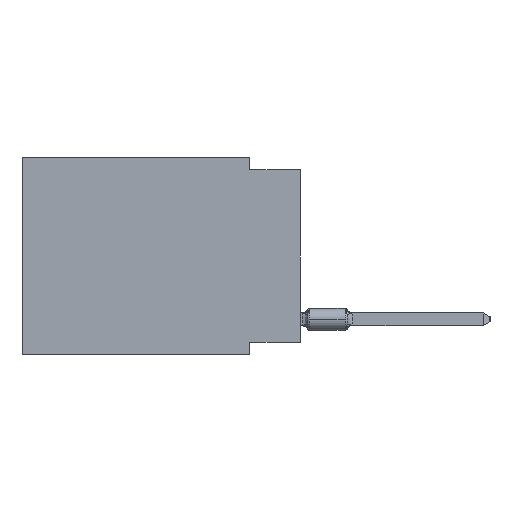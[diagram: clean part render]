
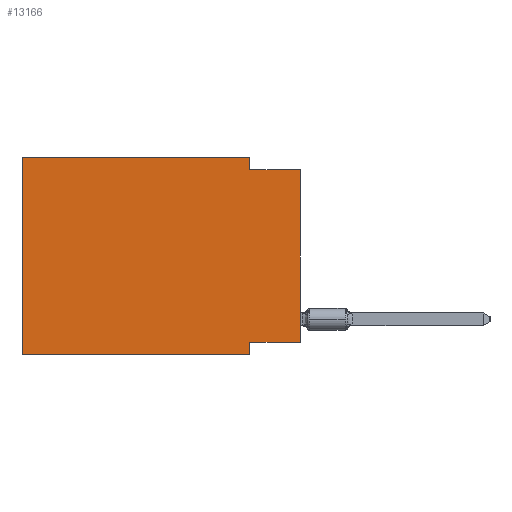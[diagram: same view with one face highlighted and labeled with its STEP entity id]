
A CAD part, left-side view. The second image highlights one B-rep face of the part: STEP entity #13166.
In plain terms, the highlighted planar face has unit normal (-1, 0, 0).
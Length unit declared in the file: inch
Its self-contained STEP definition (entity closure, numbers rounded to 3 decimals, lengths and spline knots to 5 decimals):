
#811 = CARTESIAN_POINT ( 'NONE',  ( 0., 0.1, -0.39 ) ) ;
#1030 = FACE_OUTER_BOUND ( 'NONE', #21980, .T. ) ;
#1328 = VERTEX_POINT ( 'NONE', #19792 ) ;
#1569 = CARTESIAN_POINT ( 'NONE',  ( 0., 0.55, 0. ) ) ;
#1595 = ORIENTED_EDGE ( 'NONE', *, *, #17404, .F. ) ;
#1696 = LINE ( 'NONE', #11873, #10657 ) ;
#1768 = LINE ( 'NONE', #3820, #16513 ) ;
#2016 = DIRECTION ( 'NONE',  ( 0., 1., 0. ) ) ;
#2048 = VERTEX_POINT ( 'NONE', #13201 ) ;
#2134 = VECTOR ( 'NONE', #5665, 39.37008 ) ;
#2181 = EDGE_CURVE ( 'NONE', #24167, #15423, #7977, .T. ) ;
#2816 = PLANE ( 'NONE',  #20800 ) ;
#2994 = VERTEX_POINT ( 'NONE', #12613 ) ;
#3820 = CARTESIAN_POINT ( 'NONE',  ( 0., 0., -0.365 ) ) ;
#4240 = VERTEX_POINT ( 'NONE', #15169 ) ;
#4338 = CARTESIAN_POINT ( 'NONE',  ( 0., 0.55, 0. ) ) ;
#5305 = CARTESIAN_POINT ( 'NONE',  ( 0., 0.1, -0.025 ) ) ;
#5615 = EDGE_CURVE ( 'NONE', #1328, #12173, #10484, .T. ) ;
#5665 = DIRECTION ( 'NONE',  ( 0., 0., 1. ) ) ;
#7056 = ORIENTED_EDGE ( 'NONE', *, *, #11847, .F. ) ;
#7294 = LINE ( 'NONE', #1569, #20851 ) ;
#7977 = LINE ( 'NONE', #13700, #12632 ) ;
#8468 = EDGE_CURVE ( 'NONE', #4240, #2048, #7294, .T. ) ;
#8539 = CARTESIAN_POINT ( 'NONE',  ( 0., 0.55, 0. ) ) ;
#8542 = ORIENTED_EDGE ( 'NONE', *, *, #8468, .F. ) ;
#9077 = DIRECTION ( 'NONE',  ( 0., 0., 1. ) ) ;
#9347 = CARTESIAN_POINT ( 'NONE',  ( 0., 0.1, 0. ) ) ;
#10484 = LINE ( 'NONE', #811, #14178 ) ;
#10657 = VECTOR ( 'NONE', #25076, 39.37008 ) ;
#11543 = DIRECTION ( 'NONE',  ( 0., -1., 0. ) ) ;
#11714 = ORIENTED_EDGE ( 'NONE', *, *, #12411, .T. ) ;
#11793 = ORIENTED_EDGE ( 'NONE', *, *, #21752, .F. ) ;
#11847 = EDGE_CURVE ( 'NONE', #2048, #17077, #16013, .T. ) ;
#11873 = CARTESIAN_POINT ( 'NONE',  ( 0., 0.1, 0. ) ) ;
#12047 = ORIENTED_EDGE ( 'NONE', *, *, #5615, .F. ) ;
#12173 = VERTEX_POINT ( 'NONE', #21575 ) ;
#12200 = DIRECTION ( 'NONE',  ( 0., -1., 0. ) ) ;
#12352 = CARTESIAN_POINT ( 'NONE',  ( 0., 0.55, -0.39 ) ) ;
#12411 = EDGE_CURVE ( 'NONE', #2994, #15423, #16956, .T. ) ;
#12613 = CARTESIAN_POINT ( 'NONE',  ( 0., 0., -0.365 ) ) ;
#12632 = VECTOR ( 'NONE', #11543, 39.37008 ) ;
#13166 = ADVANCED_FACE ( 'NONE', ( #1030 ), #2816, .F. ) ;
#13201 = CARTESIAN_POINT ( 'NONE',  ( 0., 0.55, 0. ) ) ;
#13700 = CARTESIAN_POINT ( 'NONE',  ( 0., 0., -0.025 ) ) ;
#14178 = VECTOR ( 'NONE', #20236, 39.37008 ) ;
#14689 = VECTOR ( 'NONE', #12200, 39.37008 ) ;
#15169 = CARTESIAN_POINT ( 'NONE',  ( 0., 0.55, -0.39 ) ) ;
#15423 = VERTEX_POINT ( 'NONE', #24628 ) ;
#15645 = ORIENTED_EDGE ( 'NONE', *, *, #2181, .F. ) ;
#15983 = ORIENTED_EDGE ( 'NONE', *, *, #22326, .T. ) ;
#16013 = LINE ( 'NONE', #4338, #14689 ) ;
#16264 = DIRECTION ( 'NONE',  ( 0., -1., 0. ) ) ;
#16420 = DIRECTION ( 'NONE',  ( 1., 0., 0. ) ) ;
#16513 = VECTOR ( 'NONE', #2016, 39.37008 ) ;
#16956 = LINE ( 'NONE', #19370, #2134 ) ;
#17077 = VERTEX_POINT ( 'NONE', #9347 ) ;
#17404 = EDGE_CURVE ( 'NONE', #2994, #1328, #1768, .T. ) ;
#19370 = CARTESIAN_POINT ( 'NONE',  ( 0., 0., 0. ) ) ;
#19792 = CARTESIAN_POINT ( 'NONE',  ( 0., 0.1, -0.365 ) ) ;
#19831 = LINE ( 'NONE', #12352, #24868 ) ;
#20236 = DIRECTION ( 'NONE',  ( 0., 0., -1. ) ) ;
#20800 = AXIS2_PLACEMENT_3D ( 'NONE', #8539, #16420, #22252 ) ;
#20851 = VECTOR ( 'NONE', #9077, 39.37008 ) ;
#21575 = CARTESIAN_POINT ( 'NONE',  ( 0., 0.1, -0.39 ) ) ;
#21752 = EDGE_CURVE ( 'NONE', #17077, #24167, #1696, .T. ) ;
#21980 = EDGE_LOOP ( 'NONE', ( #11714, #15645, #11793, #7056, #8542, #15983, #12047, #1595 ) ) ;
#22252 = DIRECTION ( 'NONE',  ( 0., 0., -1. ) ) ;
#22326 = EDGE_CURVE ( 'NONE', #4240, #12173, #19831, .T. ) ;
#24167 = VERTEX_POINT ( 'NONE', #5305 ) ;
#24628 = CARTESIAN_POINT ( 'NONE',  ( 0., 0., -0.025 ) ) ;
#24868 = VECTOR ( 'NONE', #16264, 39.37008 ) ;
#25076 = DIRECTION ( 'NONE',  ( 0., 0., -1. ) ) ;
